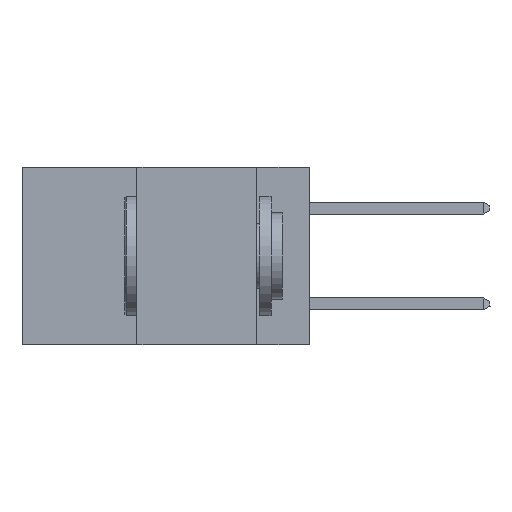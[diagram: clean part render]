
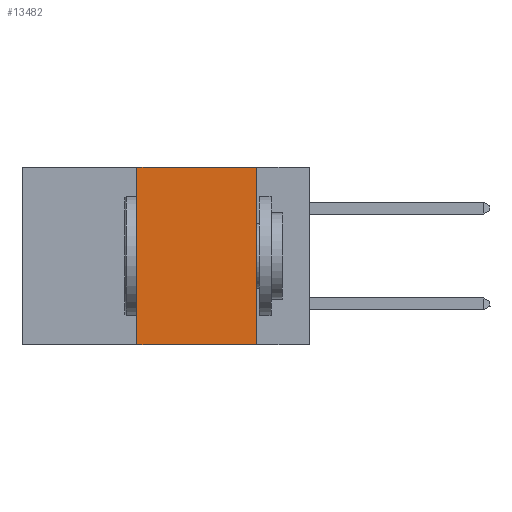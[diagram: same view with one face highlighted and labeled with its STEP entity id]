
A CAD part, left-side view. The second image highlights one B-rep face of the part: STEP entity #13482.
In plain terms, the highlighted planar face has unit normal (-1, 0, 0).
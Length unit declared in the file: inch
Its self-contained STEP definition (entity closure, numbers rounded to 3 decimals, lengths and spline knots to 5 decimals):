
#889 = CARTESIAN_POINT ( 'NONE',  ( 0., 0.36, -0.37 ) ) ;
#3368 = EDGE_CURVE ( 'NONE', #13564, #19216, #3853, .T. ) ;
#3853 = LINE ( 'NONE', #3876, #14934 ) ;
#3876 = CARTESIAN_POINT ( 'NONE',  ( 0., 0.6, 0. ) ) ;
#4356 = LINE ( 'NONE', #15360, #16231 ) ;
#5426 = VECTOR ( 'NONE', #7702, 39.37008 ) ;
#5543 = EDGE_CURVE ( 'NONE', #7416, #13564, #11782, .T. ) ;
#5684 = CARTESIAN_POINT ( 'NONE',  ( 0., 0.6, 0. ) ) ;
#6317 = VECTOR ( 'NONE', #15628, 39.37008 ) ;
#7416 = VERTEX_POINT ( 'NONE', #889 ) ;
#7702 = DIRECTION ( 'NONE',  ( 0., 0., 1. ) ) ;
#7801 = PLANE ( 'NONE',  #13417 ) ;
#8225 = ORIENTED_EDGE ( 'NONE', *, *, #29384, .F. ) ;
#10357 = DIRECTION ( 'NONE',  ( 0., 0., -1. ) ) ;
#11782 = LINE ( 'NONE', #30639, #5426 ) ;
#13417 = AXIS2_PLACEMENT_3D ( 'NONE', #5684, #21086, #31922 ) ;
#13482 = ADVANCED_FACE ( 'NONE', ( #32339 ), #7801, .F. ) ;
#13564 = VERTEX_POINT ( 'NONE', #31157 ) ;
#14934 = VECTOR ( 'NONE', #21724, 39.37008 ) ;
#15360 = CARTESIAN_POINT ( 'NONE',  ( 0., 0.11, 0. ) ) ;
#15628 = DIRECTION ( 'NONE',  ( 0., -1., 0. ) ) ;
#16231 = VECTOR ( 'NONE', #10357, 39.37008 ) ;
#17570 = VERTEX_POINT ( 'NONE', #27291 ) ;
#19216 = VERTEX_POINT ( 'NONE', #30946 ) ;
#20041 = EDGE_CURVE ( 'NONE', #7416, #17570, #23095, .T. ) ;
#21086 = DIRECTION ( 'NONE',  ( 1., 0., 0. ) ) ;
#21724 = DIRECTION ( 'NONE',  ( 0., -1., 0. ) ) ;
#22766 = EDGE_LOOP ( 'NONE', ( #8225, #25504, #26419, #32958 ) ) ;
#23095 = LINE ( 'NONE', #31026, #6317 ) ;
#25504 = ORIENTED_EDGE ( 'NONE', *, *, #3368, .F. ) ;
#26419 = ORIENTED_EDGE ( 'NONE', *, *, #5543, .F. ) ;
#27291 = CARTESIAN_POINT ( 'NONE',  ( 0., 0.11, -0.37 ) ) ;
#29384 = EDGE_CURVE ( 'NONE', #19216, #17570, #4356, .T. ) ;
#30639 = CARTESIAN_POINT ( 'NONE',  ( 0., 0.36, 0. ) ) ;
#30946 = CARTESIAN_POINT ( 'NONE',  ( 0., 0.11, 0. ) ) ;
#31026 = CARTESIAN_POINT ( 'NONE',  ( 0., 0.6, -0.37 ) ) ;
#31157 = CARTESIAN_POINT ( 'NONE',  ( 0., 0.36, 0. ) ) ;
#31922 = DIRECTION ( 'NONE',  ( 0., 0., -1. ) ) ;
#32339 = FACE_OUTER_BOUND ( 'NONE', #22766, .T. ) ;
#32958 = ORIENTED_EDGE ( 'NONE', *, *, #20041, .T. ) ;
